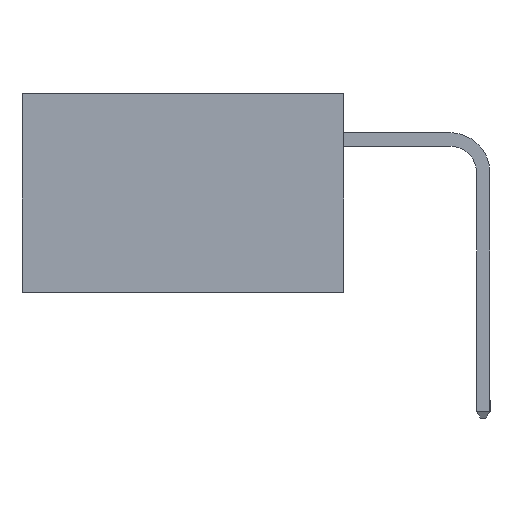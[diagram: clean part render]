
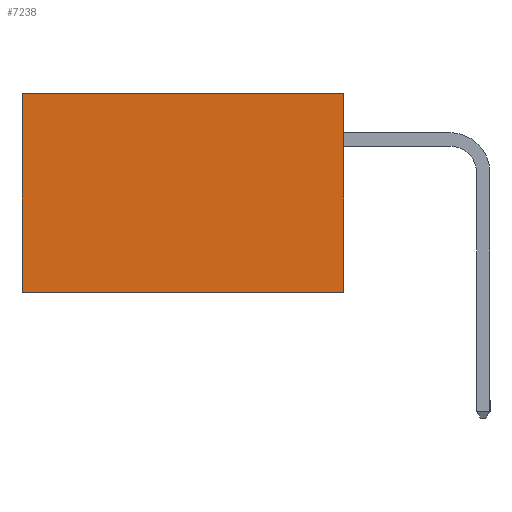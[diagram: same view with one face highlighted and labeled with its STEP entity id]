
A CAD part, left-side view. The second image highlights one B-rep face of the part: STEP entity #7238.
In plain terms, the highlighted planar face has unit normal (-1, 0, 0).
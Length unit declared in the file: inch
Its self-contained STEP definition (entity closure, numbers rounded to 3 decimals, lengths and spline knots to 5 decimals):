
#262 = VERTEX_POINT ( 'NONE', #3116 ) ;
#460 = VERTEX_POINT ( 'NONE', #11860 ) ;
#592 = CARTESIAN_POINT ( 'NONE',  ( 0.2615, 0.6, -0.37 ) ) ;
#1365 = CARTESIAN_POINT ( 'NONE',  ( 0.2615, 0.6, 0. ) ) ;
#2305 = CARTESIAN_POINT ( 'NONE',  ( 0.2615, 0., -0.37 ) ) ;
#2983 = EDGE_CURVE ( 'NONE', #460, #8950, #14075, .T. ) ;
#3079 = ORIENTED_EDGE ( 'NONE', *, *, #9151, .F. ) ;
#3116 = CARTESIAN_POINT ( 'NONE',  ( 0.2615, 0., 0. ) ) ;
#3491 = DIRECTION ( 'NONE',  ( 0., 0., -1. ) ) ;
#3865 = DIRECTION ( 'NONE',  ( 0., 1., 0. ) ) ;
#4631 = PLANE ( 'NONE',  #6419 ) ;
#5005 = FACE_OUTER_BOUND ( 'NONE', #11304, .T. ) ;
#5368 = DIRECTION ( 'NONE',  ( 0., 1., 0. ) ) ;
#5915 = DIRECTION ( 'NONE',  ( 1., 0., 0. ) ) ;
#6118 = ORIENTED_EDGE ( 'NONE', *, *, #14578, .T. ) ;
#6336 = CARTESIAN_POINT ( 'NONE',  ( 0.2615, 0.6, -0.37 ) ) ;
#6401 = LINE ( 'NONE', #11040, #9577 ) ;
#6419 = AXIS2_PLACEMENT_3D ( 'NONE', #12907, #5915, #14039 ) ;
#6812 = EDGE_CURVE ( 'NONE', #11215, #8950, #8250, .T. ) ;
#7238 = ADVANCED_FACE ( 'NONE', ( #5005 ), #4631, .F. ) ;
#7593 = ORIENTED_EDGE ( 'NONE', *, *, #6812, .T. ) ;
#8250 = LINE ( 'NONE', #6336, #10979 ) ;
#8561 = ORIENTED_EDGE ( 'NONE', *, *, #2983, .F. ) ;
#8950 = VERTEX_POINT ( 'NONE', #592 ) ;
#8984 = LINE ( 'NONE', #15174, #13981 ) ;
#9151 = EDGE_CURVE ( 'NONE', #262, #460, #8984, .T. ) ;
#9577 = VECTOR ( 'NONE', #3865, 39.37008 ) ;
#10979 = VECTOR ( 'NONE', #12227, 39.37008 ) ;
#11040 = CARTESIAN_POINT ( 'NONE',  ( 0.2615, 0., 0. ) ) ;
#11080 = VECTOR ( 'NONE', #5368, 39.37008 ) ;
#11215 = VERTEX_POINT ( 'NONE', #1365 ) ;
#11304 = EDGE_LOOP ( 'NONE', ( #7593, #8561, #3079, #6118 ) ) ;
#11860 = CARTESIAN_POINT ( 'NONE',  ( 0.2615, 0., -0.37 ) ) ;
#12227 = DIRECTION ( 'NONE',  ( 0., 0., -1. ) ) ;
#12907 = CARTESIAN_POINT ( 'NONE',  ( 0.2615, 0., -0.37 ) ) ;
#13981 = VECTOR ( 'NONE', #3491, 39.37008 ) ;
#14039 = DIRECTION ( 'NONE',  ( 0., 0., -1. ) ) ;
#14075 = LINE ( 'NONE', #2305, #11080 ) ;
#14578 = EDGE_CURVE ( 'NONE', #262, #11215, #6401, .T. ) ;
#15174 = CARTESIAN_POINT ( 'NONE',  ( 0.2615, 0., -0.37 ) ) ;
